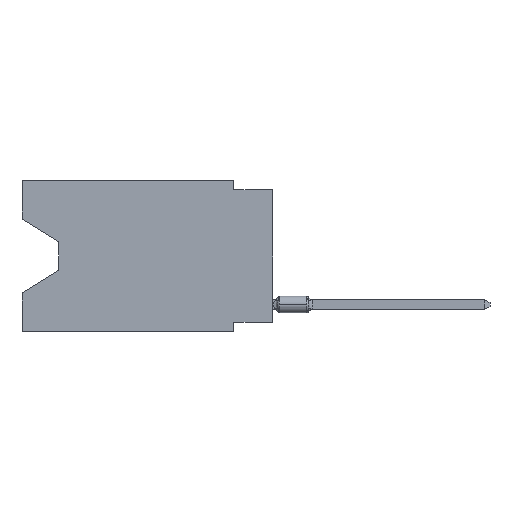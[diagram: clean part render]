
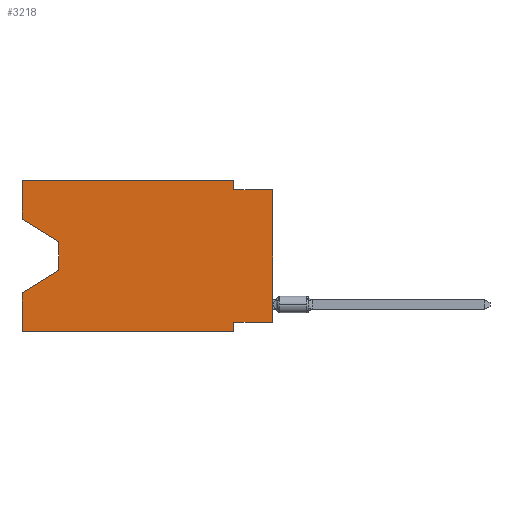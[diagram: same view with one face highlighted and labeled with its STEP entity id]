
A CAD part, left-side view. The second image highlights one B-rep face of the part: STEP entity #3218.
In plain terms, the highlighted planar face has unit normal (-1, 0, 0).
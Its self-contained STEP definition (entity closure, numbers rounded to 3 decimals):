
#55 = LINE ( 'NONE', #15399, #14895 ) ;
#70 = DIRECTION ( 'NONE',  ( 0., 1., 0. ) ) ;
#338 = VECTOR ( 'NONE', #14272, 1000. ) ;
#426 = CARTESIAN_POINT ( 'NONE',  ( 0., 13.97, -5.893 ) ) ;
#529 = CARTESIAN_POINT ( 'NONE',  ( 0., 16.383, 0. ) ) ;
#570 = LINE ( 'NONE', #4515, #7593 ) ;
#696 = VERTEX_POINT ( 'NONE', #9337 ) ;
#1748 = VERTEX_POINT ( 'NONE', #3460 ) ;
#1749 = CARTESIAN_POINT ( 'NONE',  ( 0., 2.54, -9.906 ) ) ;
#2182 = ORIENTED_EDGE ( 'NONE', *, *, #4000, .F. ) ;
#2274 = EDGE_LOOP ( 'NONE', ( #7989, #9672, #13113, #10179, #5723, #5331, #15186, #10098, #14592, #9979, #8994, #2182 ) ) ;
#2445 = CARTESIAN_POINT ( 'NONE',  ( 0., 16.383, 0. ) ) ;
#2770 = VERTEX_POINT ( 'NONE', #11412 ) ;
#2842 = DIRECTION ( 'NONE',  ( 0., 0., 1. ) ) ;
#2970 = FACE_OUTER_BOUND ( 'NONE', #2274, .T. ) ;
#3131 = LINE ( 'NONE', #14039, #4934 ) ;
#3218 = ADVANCED_FACE ( 'NONE', ( #2970 ), #5494, .F. ) ;
#3253 = LINE ( 'NONE', #6794, #9897 ) ;
#3275 = DIRECTION ( 'NONE',  ( 0., 0.855, -0.519 ) ) ;
#3294 = CARTESIAN_POINT ( 'NONE',  ( 0., 2.54, -0.635 ) ) ;
#3322 = EDGE_CURVE ( 'NONE', #1748, #7647, #14199, .T. ) ;
#3328 = DIRECTION ( 'NONE',  ( 0., 0., -1. ) ) ;
#3460 = CARTESIAN_POINT ( 'NONE',  ( 0., 16.383, -2.546 ) ) ;
#3733 = VERTEX_POINT ( 'NONE', #10643 ) ;
#3950 = VECTOR ( 'NONE', #11372, 1000. ) ;
#4000 = EDGE_CURVE ( 'NONE', #1748, #12814, #9888, .T. ) ;
#4080 = VERTEX_POINT ( 'NONE', #5108 ) ;
#4098 = VECTOR ( 'NONE', #2842, 1000. ) ;
#4115 = VERTEX_POINT ( 'NONE', #13501 ) ;
#4403 = VECTOR ( 'NONE', #9223, 1000. ) ;
#4447 = DIRECTION ( 'NONE',  ( 0., -1., 0. ) ) ;
#4515 = CARTESIAN_POINT ( 'NONE',  ( 0., 2.54, 0. ) ) ;
#4544 = CARTESIAN_POINT ( 'NONE',  ( 0., 16.383, -2.546 ) ) ;
#4633 = EDGE_CURVE ( 'NONE', #2770, #4984, #570, .T. ) ;
#4934 = VECTOR ( 'NONE', #11235, 1000. ) ;
#4984 = VERTEX_POINT ( 'NONE', #3294 ) ;
#5108 = CARTESIAN_POINT ( 'NONE',  ( 0., 16.383, -7.36 ) ) ;
#5330 = DIRECTION ( 'NONE',  ( 1., 0., 0. ) ) ;
#5331 = ORIENTED_EDGE ( 'NONE', *, *, #14393, .F. ) ;
#5425 = EDGE_CURVE ( 'NONE', #9651, #4080, #11045, .T. ) ;
#5494 = PLANE ( 'NONE',  #6623 ) ;
#5723 = ORIENTED_EDGE ( 'NONE', *, *, #13831, .T. ) ;
#6477 = EDGE_CURVE ( 'NONE', #4115, #9624, #10839, .T. ) ;
#6623 = AXIS2_PLACEMENT_3D ( 'NONE', #529, #5330, #7845 ) ;
#6794 = CARTESIAN_POINT ( 'NONE',  ( 0., 0., -0.635 ) ) ;
#7063 = VECTOR ( 'NONE', #70, 1000. ) ;
#7400 = VECTOR ( 'NONE', #9736, 1000. ) ;
#7493 = CARTESIAN_POINT ( 'NONE',  ( 0., 16.383, -9.906 ) ) ;
#7593 = VECTOR ( 'NONE', #3328, 1000. ) ;
#7622 = LINE ( 'NONE', #15007, #3950 ) ;
#7635 = EDGE_CURVE ( 'NONE', #7647, #9651, #7622, .T. ) ;
#7647 = VERTEX_POINT ( 'NONE', #11290 ) ;
#7845 = DIRECTION ( 'NONE',  ( 0., 0., -1. ) ) ;
#7989 = ORIENTED_EDGE ( 'NONE', *, *, #3322, .T. ) ;
#8070 = CARTESIAN_POINT ( 'NONE',  ( 0., 13.97, -5.893 ) ) ;
#8178 = DIRECTION ( 'NONE',  ( 0., 0., -1. ) ) ;
#8192 = CARTESIAN_POINT ( 'NONE',  ( 0., 0., -9.271 ) ) ;
#8557 = EDGE_CURVE ( 'NONE', #4984, #3733, #3253, .T. ) ;
#8597 = EDGE_CURVE ( 'NONE', #12814, #2770, #9058, .T. ) ;
#8666 = LINE ( 'NONE', #11247, #4098 ) ;
#8683 = CARTESIAN_POINT ( 'NONE',  ( 0., 2.54, -9.271 ) ) ;
#8988 = CARTESIAN_POINT ( 'NONE',  ( 0., 16.383, 0. ) ) ;
#8994 = ORIENTED_EDGE ( 'NONE', *, *, #8597, .F. ) ;
#9058 = LINE ( 'NONE', #8988, #4403 ) ;
#9223 = DIRECTION ( 'NONE',  ( 0., -1., 0. ) ) ;
#9337 = CARTESIAN_POINT ( 'NONE',  ( 0., 16.383, -9.906 ) ) ;
#9624 = VERTEX_POINT ( 'NONE', #8683 ) ;
#9651 = VERTEX_POINT ( 'NONE', #426 ) ;
#9672 = ORIENTED_EDGE ( 'NONE', *, *, #7635, .T. ) ;
#9736 = DIRECTION ( 'NONE',  ( 0., 0., 1. ) ) ;
#9888 = LINE ( 'NONE', #2445, #7400 ) ;
#9897 = VECTOR ( 'NONE', #4447, 1000. ) ;
#9899 = EDGE_CURVE ( 'NONE', #696, #4080, #3131, .T. ) ;
#9979 = ORIENTED_EDGE ( 'NONE', *, *, #4633, .F. ) ;
#10098 = ORIENTED_EDGE ( 'NONE', *, *, #13772, .T. ) ;
#10179 = ORIENTED_EDGE ( 'NONE', *, *, #9899, .F. ) ;
#10643 = CARTESIAN_POINT ( 'NONE',  ( 0., 0., -0.635 ) ) ;
#10839 = LINE ( 'NONE', #8192, #7063 ) ;
#11045 = LINE ( 'NONE', #8070, #13302 ) ;
#11235 = DIRECTION ( 'NONE',  ( 0., 0., 1. ) ) ;
#11247 = CARTESIAN_POINT ( 'NONE',  ( 0., 0., 0. ) ) ;
#11290 = CARTESIAN_POINT ( 'NONE',  ( 0., 13.97, -4.013 ) ) ;
#11346 = VECTOR ( 'NONE', #12265, 1000. ) ;
#11372 = DIRECTION ( 'NONE',  ( 0., 0., -1. ) ) ;
#11412 = CARTESIAN_POINT ( 'NONE',  ( 0., 2.54, 0. ) ) ;
#12131 = CARTESIAN_POINT ( 'NONE',  ( 0., 16.383, 0. ) ) ;
#12265 = DIRECTION ( 'NONE',  ( 0., -1., 0. ) ) ;
#12814 = VERTEX_POINT ( 'NONE', #12131 ) ;
#13113 = ORIENTED_EDGE ( 'NONE', *, *, #5425, .T. ) ;
#13302 = VECTOR ( 'NONE', #3275, 1000. ) ;
#13501 = CARTESIAN_POINT ( 'NONE',  ( 0., 0., -9.271 ) ) ;
#13772 = EDGE_CURVE ( 'NONE', #4115, #3733, #8666, .T. ) ;
#13819 = VERTEX_POINT ( 'NONE', #1749 ) ;
#13831 = EDGE_CURVE ( 'NONE', #696, #13819, #14628, .T. ) ;
#14039 = CARTESIAN_POINT ( 'NONE',  ( 0., 16.383, 0. ) ) ;
#14199 = LINE ( 'NONE', #4544, #338 ) ;
#14272 = DIRECTION ( 'NONE',  ( 0., -0.855, -0.519 ) ) ;
#14393 = EDGE_CURVE ( 'NONE', #9624, #13819, #55, .T. ) ;
#14592 = ORIENTED_EDGE ( 'NONE', *, *, #8557, .F. ) ;
#14628 = LINE ( 'NONE', #7493, #11346 ) ;
#14895 = VECTOR ( 'NONE', #8178, 1000. ) ;
#15007 = CARTESIAN_POINT ( 'NONE',  ( 0., 13.97, -4.013 ) ) ;
#15186 = ORIENTED_EDGE ( 'NONE', *, *, #6477, .F. ) ;
#15399 = CARTESIAN_POINT ( 'NONE',  ( 0., 2.54, -9.906 ) ) ;
